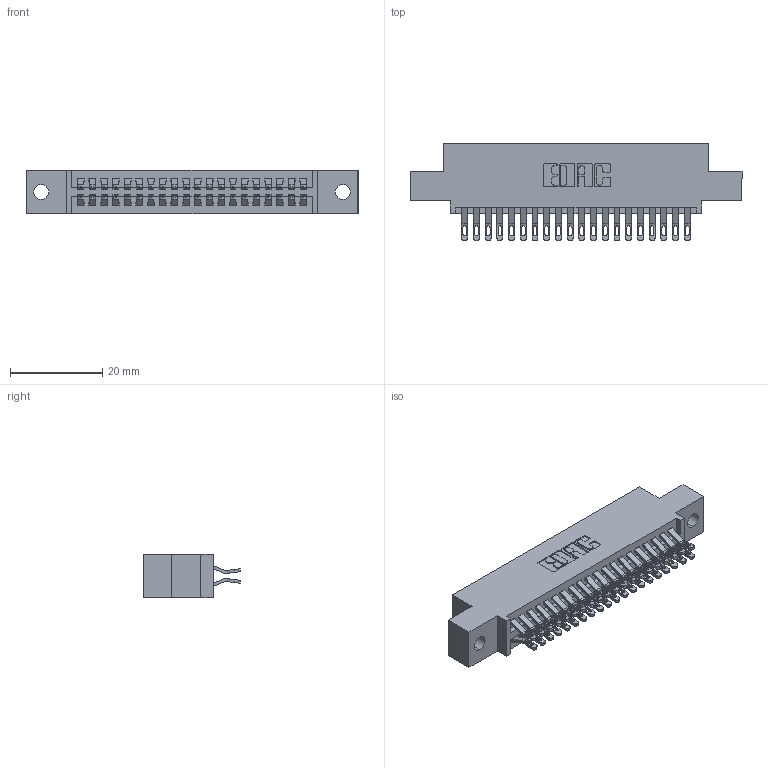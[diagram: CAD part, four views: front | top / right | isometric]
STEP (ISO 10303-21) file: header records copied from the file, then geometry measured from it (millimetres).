
FILE_DESCRIPTION (( 'STEP AP203' ), '1' );
FILE_NAME ('345-040-555-502.STEP', '2018-09-05T04:52:07', ( '' ), ( '' ), 'SwSTEP 2.0', 'SolidWorks 2016', '' );
FILE_SCHEMA (( 'CONFIG_CONTROL_DESIGN' ));
Length unit declared in the file: inch
Products named in the file (3): 345 Part_0.110 Offset - 0.128 Dia; 345-292-001_555 Tail; 345-040-555-502
Assembly tree (41 placements, depth 2):
  345-040-555-502
    345 Part_0.110 Offset - 0.128 Dia
    345-292-001_555 Tail  x40
Bounding box: 72.01 x 21.13 x 9.4 mm (x, y, z)
Volume: 6796.8 mm3; surface area: 9844.3 mm2
Topology: 41 solids, 41 shells, 2370 faces, 7433 edges, 4954 vertices
Faces by surface type: plane 1324, cylinder 1046
Entity records: 19115 total; most frequent: CARTESIAN_POINT 3262, ORIENTED_EDGE 3166, DIRECTION 2871, EDGE_CURVE 1583, VECTOR 1351, LINE 1351, VERTEX_POINT 1054, AXIS2_PLACEMENT_3D 760
